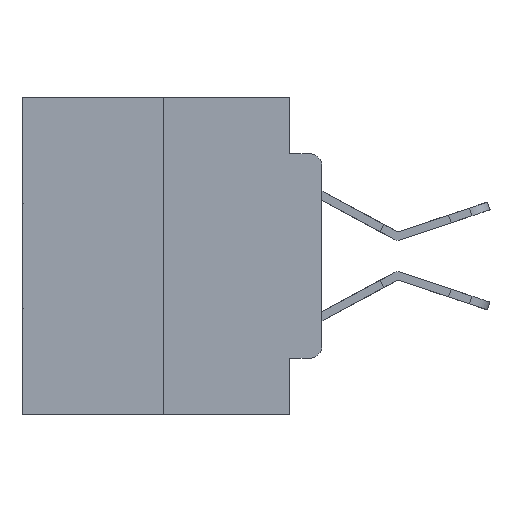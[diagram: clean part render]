
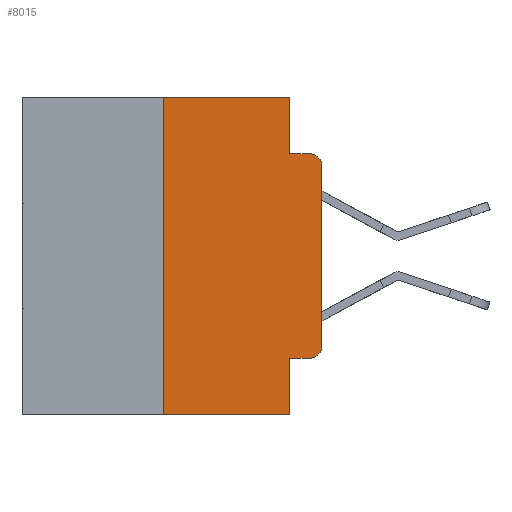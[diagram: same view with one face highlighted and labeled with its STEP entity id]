
A CAD part, left-side view. The second image highlights one B-rep face of the part: STEP entity #8015.
In plain terms, the highlighted planar face has unit normal (-1, 0, 0).
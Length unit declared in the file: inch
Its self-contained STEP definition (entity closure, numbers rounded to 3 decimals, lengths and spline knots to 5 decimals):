
#34 = FACE_OUTER_BOUND ( 'NONE', #10761, .T. ) ;
#460 = EDGE_CURVE ( 'NONE', #28826, #14637, #11332, .T. ) ;
#822 = DIRECTION ( 'NONE',  ( 0., 0., -1. ) ) ;
#1093 = VERTEX_POINT ( 'NONE', #25440 ) ;
#2119 = LINE ( 'NONE', #26947, #7740 ) ;
#2159 = EDGE_CURVE ( 'NONE', #7863, #1093, #6758, .T. ) ;
#2836 = DIRECTION ( 'NONE',  ( 0., -1., 0. ) ) ;
#3875 = ORIENTED_EDGE ( 'NONE', *, *, #25938, .T. ) ;
#4034 = CARTESIAN_POINT ( 'NONE',  ( 0., 0.051, 0. ) ) ;
#4092 = EDGE_CURVE ( 'NONE', #20287, #14637, #16975, .T. ) ;
#5148 = ORIENTED_EDGE ( 'NONE', *, *, #4092, .T. ) ;
#5247 = LINE ( 'NONE', #8805, #29205 ) ;
#5419 = VERTEX_POINT ( 'NONE', #21523 ) ;
#5564 = CARTESIAN_POINT ( 'NONE',  ( 0., 0.051, 0. ) ) ;
#5673 = CARTESIAN_POINT ( 'NONE',  ( 0., 0., -0.1085 ) ) ;
#5796 = ORIENTED_EDGE ( 'NONE', *, *, #460, .F. ) ;
#6071 = EDGE_CURVE ( 'NONE', #8832, #13258, #25151, .T. ) ;
#6750 = DIRECTION ( 'NONE',  ( 0., 0., -1. ) ) ;
#6758 = LINE ( 'NONE', #14468, #29943 ) ;
#6878 = CARTESIAN_POINT ( 'NONE',  ( 0., 0.25, 0. ) ) ;
#6922 = CARTESIAN_POINT ( 'NONE',  ( 0., 0.02, -0.0885 ) ) ;
#7008 = VERTEX_POINT ( 'NONE', #8654 ) ;
#7101 = ORIENTED_EDGE ( 'NONE', *, *, #25844, .F. ) ;
#7740 = VECTOR ( 'NONE', #29199, 39.37008 ) ;
#7755 = ORIENTED_EDGE ( 'NONE', *, *, #6071, .F. ) ;
#7762 = ORIENTED_EDGE ( 'NONE', *, *, #8212, .T. ) ;
#7863 = VERTEX_POINT ( 'NONE', #15685 ) ;
#8015 = ADVANCED_FACE ( 'NONE', ( #34 ), #16165, .F. ) ;
#8212 = EDGE_CURVE ( 'NONE', #1093, #7008, #10903, .T. ) ;
#8539 = ORIENTED_EDGE ( 'NONE', *, *, #22387, .F. ) ;
#8654 = CARTESIAN_POINT ( 'NONE',  ( 0., 0., -0.3915 ) ) ;
#8805 = CARTESIAN_POINT ( 'NONE',  ( 0., 0.473, -0.5 ) ) ;
#8832 = VERTEX_POINT ( 'NONE', #19096 ) ;
#9882 = DIRECTION ( 'NONE',  ( -1., 0., 0. ) ) ;
#10761 = EDGE_LOOP ( 'NONE', ( #3875, #5148, #5796, #7101, #7755, #8539, #10793, #22687, #13044, #7762 ) ) ;
#10793 = ORIENTED_EDGE ( 'NONE', *, *, #15176, .T. ) ;
#10903 = CIRCLE ( 'NONE', #30108, 0.02 ) ;
#11332 = LINE ( 'NONE', #20626, #24348 ) ;
#12218 = LINE ( 'NONE', #5564, #17656 ) ;
#12297 = DIRECTION ( 'NONE',  ( -1., 0., 0. ) ) ;
#12899 = VECTOR ( 'NONE', #2836, 39.37008 ) ;
#13044 = ORIENTED_EDGE ( 'NONE', *, *, #2159, .T. ) ;
#13258 = VERTEX_POINT ( 'NONE', #22670 ) ;
#13760 = CARTESIAN_POINT ( 'NONE',  ( 0., 0.25, -0.5 ) ) ;
#14098 = DIRECTION ( 'NONE',  ( 0., -1., 0. ) ) ;
#14468 = CARTESIAN_POINT ( 'NONE',  ( 0., 0.051, -0.4115 ) ) ;
#14637 = VERTEX_POINT ( 'NONE', #6922 ) ;
#15176 = EDGE_CURVE ( 'NONE', #28500, #5419, #5247, .T. ) ;
#15685 = CARTESIAN_POINT ( 'NONE',  ( 0., 0.051, -0.4115 ) ) ;
#15954 = LINE ( 'NONE', #6878, #27417 ) ;
#16165 = PLANE ( 'NONE',  #16335 ) ;
#16335 = AXIS2_PLACEMENT_3D ( 'NONE', #18433, #20743, #6750 ) ;
#16975 = CIRCLE ( 'NONE', #19111, 0.02 ) ;
#17656 = VECTOR ( 'NONE', #822, 39.37008 ) ;
#18088 = DIRECTION ( 'NONE',  ( 0., -1., 0. ) ) ;
#18105 = DIRECTION ( 'NONE',  ( 0., 0., -1. ) ) ;
#18433 = CARTESIAN_POINT ( 'NONE',  ( 0., 0.473, 0. ) ) ;
#19096 = CARTESIAN_POINT ( 'NONE',  ( 0., 0.25, 0. ) ) ;
#19111 = AXIS2_PLACEMENT_3D ( 'NONE', #26103, #12297, #28383 ) ;
#20287 = VERTEX_POINT ( 'NONE', #5673 ) ;
#20626 = CARTESIAN_POINT ( 'NONE',  ( 0., 0.051, -0.0885 ) ) ;
#20743 = DIRECTION ( 'NONE',  ( 1., 0., 0. ) ) ;
#21347 = DIRECTION ( 'NONE',  ( 0., -1., 0. ) ) ;
#21523 = CARTESIAN_POINT ( 'NONE',  ( 0., 0.051, -0.5 ) ) ;
#21687 = LINE ( 'NONE', #4034, #27806 ) ;
#22387 = EDGE_CURVE ( 'NONE', #28500, #8832, #15954, .T. ) ;
#22670 = CARTESIAN_POINT ( 'NONE',  ( 0., 0.051, 0. ) ) ;
#22687 = ORIENTED_EDGE ( 'NONE', *, *, #23526, .F. ) ;
#23182 = DIRECTION ( 'NONE',  ( 0., 0., 1. ) ) ;
#23526 = EDGE_CURVE ( 'NONE', #7863, #5419, #21687, .T. ) ;
#23767 = CARTESIAN_POINT ( 'NONE',  ( 0., 0.02, -0.3915 ) ) ;
#24079 = CARTESIAN_POINT ( 'NONE',  ( 0., 0.051, -0.0885 ) ) ;
#24348 = VECTOR ( 'NONE', #14098, 39.37008 ) ;
#25151 = LINE ( 'NONE', #28427, #12899 ) ;
#25440 = CARTESIAN_POINT ( 'NONE',  ( 0., 0.02, -0.4115 ) ) ;
#25844 = EDGE_CURVE ( 'NONE', #13258, #28826, #12218, .T. ) ;
#25938 = EDGE_CURVE ( 'NONE', #7008, #20287, #2119, .T. ) ;
#26086 = DIRECTION ( 'NONE',  ( 0., 0., -1. ) ) ;
#26103 = CARTESIAN_POINT ( 'NONE',  ( 0., 0.02, -0.1085 ) ) ;
#26947 = CARTESIAN_POINT ( 'NONE',  ( 0., 0., 0. ) ) ;
#27417 = VECTOR ( 'NONE', #23182, 39.37008 ) ;
#27806 = VECTOR ( 'NONE', #18105, 39.37008 ) ;
#28383 = DIRECTION ( 'NONE',  ( 0., 0., -1. ) ) ;
#28427 = CARTESIAN_POINT ( 'NONE',  ( 0., 0.473, 0. ) ) ;
#28500 = VERTEX_POINT ( 'NONE', #13760 ) ;
#28826 = VERTEX_POINT ( 'NONE', #24079 ) ;
#29199 = DIRECTION ( 'NONE',  ( 0., 0., 1. ) ) ;
#29205 = VECTOR ( 'NONE', #18088, 39.37008 ) ;
#29943 = VECTOR ( 'NONE', #21347, 39.37008 ) ;
#30108 = AXIS2_PLACEMENT_3D ( 'NONE', #23767, #9882, #26086 ) ;
